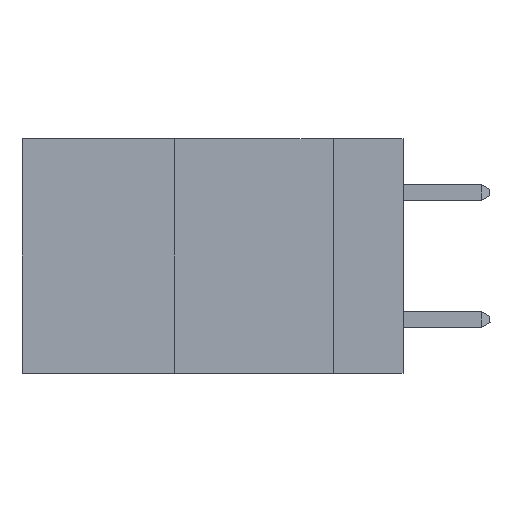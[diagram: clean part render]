
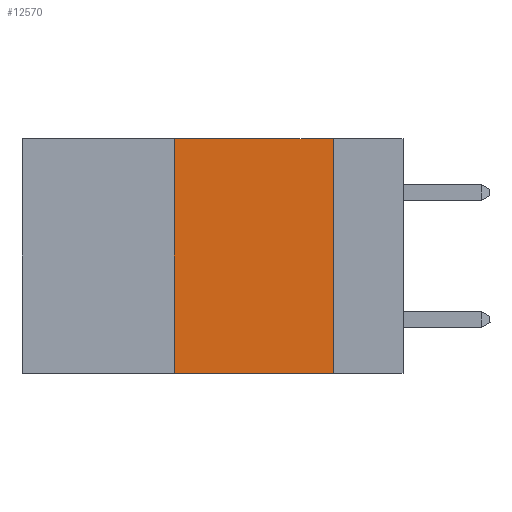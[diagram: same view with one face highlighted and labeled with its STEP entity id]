
A CAD part, left-side view. The second image highlights one B-rep face of the part: STEP entity #12570.
In plain terms, the highlighted planar face has unit normal (-1, 0, 0).
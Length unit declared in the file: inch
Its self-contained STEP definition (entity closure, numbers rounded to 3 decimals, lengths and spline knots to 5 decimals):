
#967 = CARTESIAN_POINT ( 'NONE',  ( 0., 0.6, -0.37 ) ) ;
#1115 = VECTOR ( 'NONE', #13648, 39.37008 ) ;
#3918 = VECTOR ( 'NONE', #15972, 39.37008 ) ;
#4211 = DIRECTION ( 'NONE',  ( 0., 0., -1. ) ) ;
#5040 = FACE_OUTER_BOUND ( 'NONE', #9842, .T. ) ;
#5331 = CARTESIAN_POINT ( 'NONE',  ( 0., 0.6, 0. ) ) ;
#5553 = EDGE_CURVE ( 'NONE', #15009, #9310, #15307, .T. ) ;
#6079 = ORIENTED_EDGE ( 'NONE', *, *, #9206, .F. ) ;
#6377 = EDGE_CURVE ( 'NONE', #12750, #18249, #7963, .T. ) ;
#6548 = ORIENTED_EDGE ( 'NONE', *, *, #17035, .F. ) ;
#6562 = LINE ( 'NONE', #12925, #17811 ) ;
#7828 = CARTESIAN_POINT ( 'NONE',  ( 0., 0.11, 0. ) ) ;
#7963 = LINE ( 'NONE', #967, #3918 ) ;
#8684 = CARTESIAN_POINT ( 'NONE',  ( 0., 0.6, 0. ) ) ;
#8771 = CARTESIAN_POINT ( 'NONE',  ( 0., 0.11, 0. ) ) ;
#9206 = EDGE_CURVE ( 'NONE', #12750, #15009, #6562, .T. ) ;
#9310 = VERTEX_POINT ( 'NONE', #8771 ) ;
#9842 = EDGE_LOOP ( 'NONE', ( #6548, #15467, #6079, #13879 ) ) ;
#10609 = CARTESIAN_POINT ( 'NONE',  ( 0., 0.36, -0.37 ) ) ;
#10893 = CARTESIAN_POINT ( 'NONE',  ( 0., 0.11, -0.37 ) ) ;
#12570 = ADVANCED_FACE ( 'NONE', ( #5040 ), #17445, .F. ) ;
#12750 = VERTEX_POINT ( 'NONE', #10609 ) ;
#12925 = CARTESIAN_POINT ( 'NONE',  ( 0., 0.36, 0. ) ) ;
#13086 = DIRECTION ( 'NONE',  ( 1., 0., 0. ) ) ;
#13395 = CARTESIAN_POINT ( 'NONE',  ( 0., 0.36, 0. ) ) ;
#13488 = AXIS2_PLACEMENT_3D ( 'NONE', #8684, #13086, #4211 ) ;
#13648 = DIRECTION ( 'NONE',  ( 0., 0., -1. ) ) ;
#13879 = ORIENTED_EDGE ( 'NONE', *, *, #6377, .T. ) ;
#14397 = DIRECTION ( 'NONE',  ( 0., 0., 1. ) ) ;
#15009 = VERTEX_POINT ( 'NONE', #13395 ) ;
#15307 = LINE ( 'NONE', #5331, #19219 ) ;
#15467 = ORIENTED_EDGE ( 'NONE', *, *, #5553, .F. ) ;
#15598 = DIRECTION ( 'NONE',  ( 0., -1., 0. ) ) ;
#15972 = DIRECTION ( 'NONE',  ( 0., -1., 0. ) ) ;
#16578 = LINE ( 'NONE', #7828, #1115 ) ;
#17035 = EDGE_CURVE ( 'NONE', #9310, #18249, #16578, .T. ) ;
#17445 = PLANE ( 'NONE',  #13488 ) ;
#17811 = VECTOR ( 'NONE', #14397, 39.37008 ) ;
#18249 = VERTEX_POINT ( 'NONE', #10893 ) ;
#19219 = VECTOR ( 'NONE', #15598, 39.37008 ) ;
